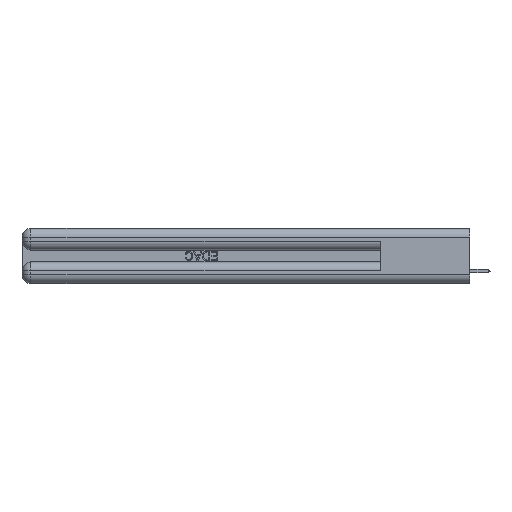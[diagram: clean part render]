
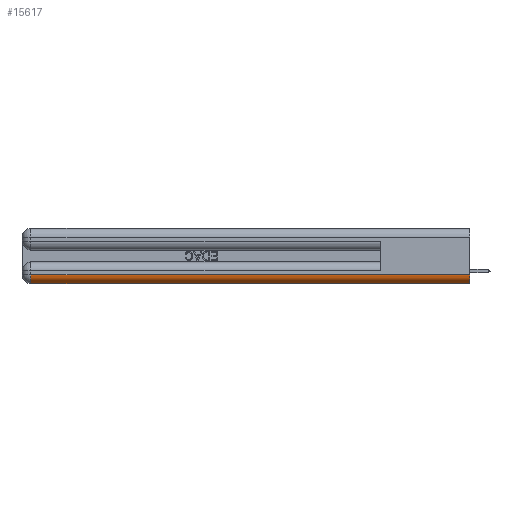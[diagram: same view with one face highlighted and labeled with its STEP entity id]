
A CAD part, left-side view. The second image highlights one B-rep face of the part: STEP entity #15617.
In plain terms, the highlighted cylindrical face has radius 1.524 mm (diameter 3.048 mm), a partial arc.
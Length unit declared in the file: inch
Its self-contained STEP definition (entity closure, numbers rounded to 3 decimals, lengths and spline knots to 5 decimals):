
#570 = ORIENTED_EDGE ( 'NONE', *, *, #45538, .F. ) ;
#2117 = VECTOR ( 'NONE', #19292, 39.37008 ) ;
#4215 = VERTEX_POINT ( 'NONE', #15414 ) ;
#4832 = ORIENTED_EDGE ( 'NONE', *, *, #20052, .F. ) ;
#5684 = ORIENTED_EDGE ( 'NONE', *, *, #29639, .F. ) ;
#10558 = CARTESIAN_POINT ( 'NONE',  ( 0.06, 0., 0.06 ) ) ;
#10572 = LINE ( 'NONE', #45083, #14421 ) ;
#14421 = VECTOR ( 'NONE', #37621, 39.37008 ) ;
#15414 = CARTESIAN_POINT ( 'NONE',  ( 0.06, 2.94, 0. ) ) ;
#15617 = ADVANCED_FACE ( 'NONE', ( #47747 ), #43201, .T. ) ;
#16930 = VERTEX_POINT ( 'NONE', #23029 ) ;
#18886 = CARTESIAN_POINT ( 'NONE',  ( 0.06, 0., 0.06 ) ) ;
#18911 = EDGE_CURVE ( 'NONE', #49385, #4215, #25970, .T. ) ;
#19035 = DIRECTION ( 'NONE',  ( 0., -1., 0. ) ) ;
#19061 = DIRECTION ( 'NONE',  ( 0., 1., 0. ) ) ;
#19292 = DIRECTION ( 'NONE',  ( 0., 1., 0. ) ) ;
#20052 = EDGE_CURVE ( 'NONE', #16930, #49385, #45313, .T. ) ;
#21949 = CARTESIAN_POINT ( 'NONE',  ( 0.06, 0., 0. ) ) ;
#23029 = CARTESIAN_POINT ( 'NONE',  ( 0., 0., 0.06 ) ) ;
#24586 = CARTESIAN_POINT ( 'NONE',  ( 0.06, 2.94, 0.06 ) ) ;
#25187 = AXIS2_PLACEMENT_3D ( 'NONE', #10558, #19035, #52066 ) ;
#25970 = LINE ( 'NONE', #49505, #2117 ) ;
#29639 = EDGE_CURVE ( 'NONE', #36842, #16930, #10572, .T. ) ;
#35821 = AXIS2_PLACEMENT_3D ( 'NONE', #18886, #19061, #47739 ) ;
#36842 = VERTEX_POINT ( 'NONE', #38431 ) ;
#37621 = DIRECTION ( 'NONE',  ( 0., -1., 0. ) ) ;
#37750 = ORIENTED_EDGE ( 'NONE', *, *, #18911, .F. ) ;
#38328 = EDGE_LOOP ( 'NONE', ( #4832, #5684, #570, #37750 ) ) ;
#38431 = CARTESIAN_POINT ( 'NONE',  ( 0., 2.94, 0.06 ) ) ;
#40636 = AXIS2_PLACEMENT_3D ( 'NONE', #24586, #45770, #49903 ) ;
#41631 = CIRCLE ( 'NONE', #40636, 0.06 ) ;
#43201 = CYLINDRICAL_SURFACE ( 'NONE', #35821, 0.06 ) ;
#45083 = CARTESIAN_POINT ( 'NONE',  ( 0., 0., 0.06 ) ) ;
#45313 = CIRCLE ( 'NONE', #25187, 0.06 ) ;
#45538 = EDGE_CURVE ( 'NONE', #4215, #36842, #41631, .T. ) ;
#45770 = DIRECTION ( 'NONE',  ( 0., 1., 0. ) ) ;
#47739 = DIRECTION ( 'NONE',  ( 0., 0., 1. ) ) ;
#47747 = FACE_OUTER_BOUND ( 'NONE', #38328, .T. ) ;
#49385 = VERTEX_POINT ( 'NONE', #21949 ) ;
#49505 = CARTESIAN_POINT ( 'NONE',  ( 0.06, 3., 0. ) ) ;
#49903 = DIRECTION ( 'NONE',  ( 0., 0., 1. ) ) ;
#52066 = DIRECTION ( 'NONE',  ( 0., 0., 1. ) ) ;
